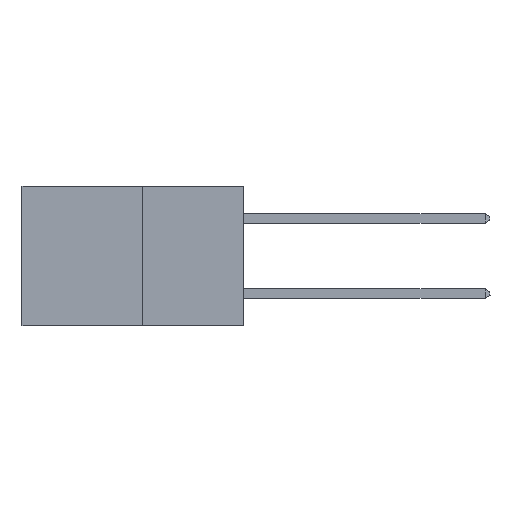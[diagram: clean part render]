
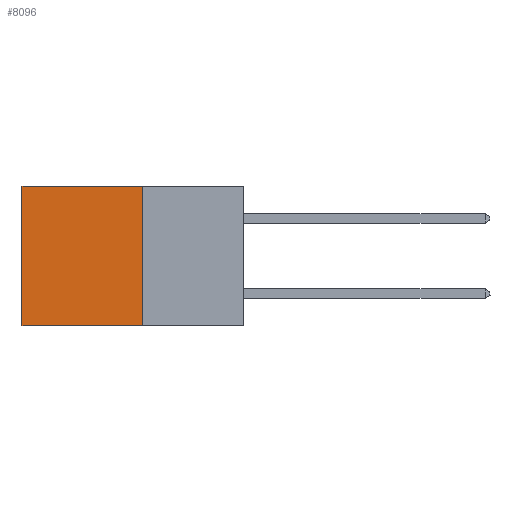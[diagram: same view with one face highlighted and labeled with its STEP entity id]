
A CAD part, left-side view. The second image highlights one B-rep face of the part: STEP entity #8096.
In plain terms, the highlighted planar face has unit normal (-1, 0, 0).
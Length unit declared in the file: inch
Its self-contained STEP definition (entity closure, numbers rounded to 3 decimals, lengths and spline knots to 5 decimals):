
#205 = EDGE_CURVE ( 'NONE', #21824, #13633, #9825, .T. ) ;
#991 = DIRECTION ( 'NONE',  ( 0., 1., 0. ) ) ;
#1705 = CARTESIAN_POINT ( 'NONE',  ( 0.277, 0.27, 0. ) ) ;
#1716 = LINE ( 'NONE', #30819, #14174 ) ;
#3423 = CARTESIAN_POINT ( 'NONE',  ( 0.277, 0.59, 0. ) ) ;
#4210 = EDGE_CURVE ( 'NONE', #17263, #21824, #1716, .T. ) ;
#4274 = ORIENTED_EDGE ( 'NONE', *, *, #205, .T. ) ;
#5702 = DIRECTION ( 'NONE',  ( 0., 0., -1. ) ) ;
#6763 = LINE ( 'NONE', #26275, #26657 ) ;
#7099 = AXIS2_PLACEMENT_3D ( 'NONE', #8082, #20649, #5702 ) ;
#7396 = LINE ( 'NONE', #20629, #20351 ) ;
#8082 = CARTESIAN_POINT ( 'NONE',  ( 0.277, 0.27, -0.37 ) ) ;
#8096 = ADVANCED_FACE ( 'NONE', ( #15546 ), #18117, .F. ) ;
#9825 = LINE ( 'NONE', #31545, #16447 ) ;
#10391 = ORIENTED_EDGE ( 'NONE', *, *, #28448, .F. ) ;
#10991 = EDGE_LOOP ( 'NONE', ( #4274, #30450, #10391, #11152 ) ) ;
#11152 = ORIENTED_EDGE ( 'NONE', *, *, #4210, .T. ) ;
#11327 = DIRECTION ( 'NONE',  ( 0., 1., 0. ) ) ;
#11693 = EDGE_CURVE ( 'NONE', #27446, #13633, #6763, .T. ) ;
#13633 = VERTEX_POINT ( 'NONE', #21159 ) ;
#14174 = VECTOR ( 'NONE', #991, 39.37008 ) ;
#15546 = FACE_OUTER_BOUND ( 'NONE', #10991, .T. ) ;
#15586 = DIRECTION ( 'NONE',  ( 0., 0., -1. ) ) ;
#16447 = VECTOR ( 'NONE', #16625, 39.37008 ) ;
#16625 = DIRECTION ( 'NONE',  ( 0., 0., -1. ) ) ;
#17263 = VERTEX_POINT ( 'NONE', #1705 ) ;
#18117 = PLANE ( 'NONE',  #7099 ) ;
#20351 = VECTOR ( 'NONE', #15586, 39.37008 ) ;
#20629 = CARTESIAN_POINT ( 'NONE',  ( 0.277, 0.27, -0.37 ) ) ;
#20649 = DIRECTION ( 'NONE',  ( 1., 0., 0. ) ) ;
#21159 = CARTESIAN_POINT ( 'NONE',  ( 0.277, 0.59, -0.37 ) ) ;
#21824 = VERTEX_POINT ( 'NONE', #3423 ) ;
#26275 = CARTESIAN_POINT ( 'NONE',  ( 0.277, 0.27, -0.37 ) ) ;
#26657 = VECTOR ( 'NONE', #11327, 39.37008 ) ;
#27446 = VERTEX_POINT ( 'NONE', #31648 ) ;
#28448 = EDGE_CURVE ( 'NONE', #17263, #27446, #7396, .T. ) ;
#30450 = ORIENTED_EDGE ( 'NONE', *, *, #11693, .F. ) ;
#30819 = CARTESIAN_POINT ( 'NONE',  ( 0.277, 0.27, 0. ) ) ;
#31545 = CARTESIAN_POINT ( 'NONE',  ( 0.277, 0.59, -0.37 ) ) ;
#31648 = CARTESIAN_POINT ( 'NONE',  ( 0.277, 0.27, -0.37 ) ) ;
